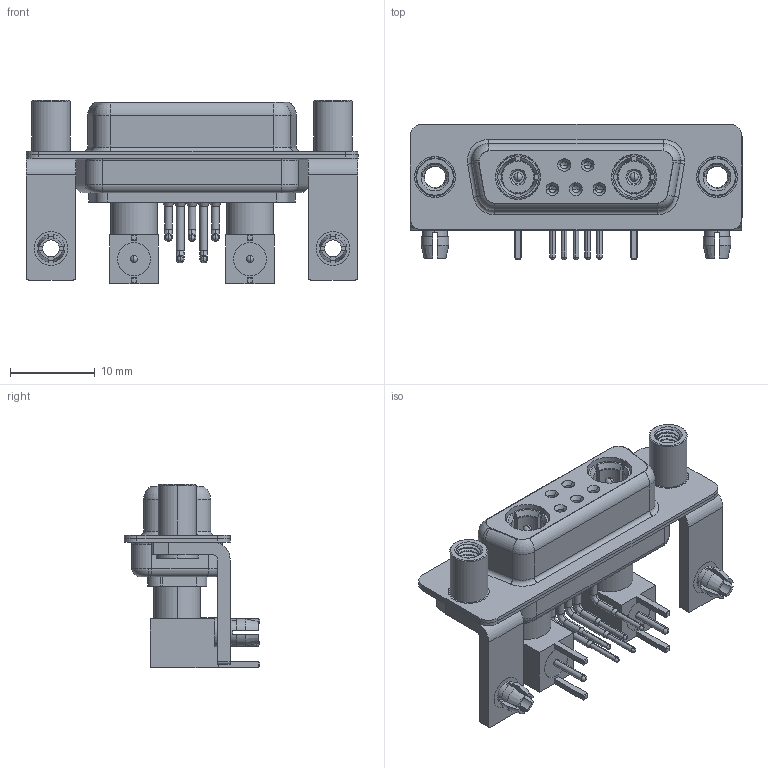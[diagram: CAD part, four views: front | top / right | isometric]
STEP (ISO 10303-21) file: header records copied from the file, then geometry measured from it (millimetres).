
FILE_DESCRIPTION (( 'STEP AP203' ), '1' );
FILE_NAME ('630-7W2-240-5ND.STEP', '2022-05-31T01:10:40', ( '' ), ( '' ), 'SwSTEP 2.0', 'SolidWorks 2020', '' );
FILE_SCHEMA (( 'CONFIG_CONTROL_DESIGN' ));
Length unit declared in the file: millimetre
Products named in the file (17): RA Back Shell; Pin_RA; Locking Collar; Insulator Pin_Straight PC Tail; Insulator RA Pin; 630Combo Contact Row 2; Co-Ax Plug Assy_RA; 630-7W2-240-5ND; 630Combo Threaded Standoff_D; 630Combo Stabilizer Bracket; Co-Ax Plug_RA PC Tail; 630Combo Shell Rear_15 Contacts; 630Combo Shell Front_15 Contacts; 630Combo Board Lock; 630Combo Housing_7W2; 630Combo Contact Row 1
Assembly tree (28 placements, depth 3):
  630-7W2-240-5ND
    630Combo Housing_7W2
    630Combo Shell Front_15 Contacts
    630Combo Shell Rear_15 Contacts
    630Combo Stabilizer Bracket  x2
    630Combo Board Lock  x2
    630Combo Threaded Standoff_D  x2
    Co-Ax Plug Assy_RA
      Co-Ax Plug_RA PC Tail
      Insulator Pin_Straight PC Tail
      Pin_RA
      Locking Collar
      RA Back Shell
      Insulator RA Pin
    Co-Ax Plug Assy_RA
      Co-Ax Plug_RA PC Tail
      Insulator Pin_Straight PC Tail
      Pin_RA
      Locking Collar
      RA Back Shell
      Insulator RA Pin
    630Combo Contact Row 1  x2
    630Combo Contact Row 2  x3
Bounding box: 39.2 x 16 x 21.61 mm (x, y, z)
Volume: 3393.1 mm3; surface area: 8460.6 mm2
Topology: 26 solids, 26 shells, 1070 faces, 2676 edges, 1692 vertices
Faces by surface type: cylinder 486, plane 346, cone 133, torus 69, bspline 28, sphere 8
Entity records: 24302 total; most frequent: CARTESIAN_POINT 6298, DIRECTION 3540, ORIENTED_EDGE 3216, EDGE_CURVE 1608, AXIS2_PLACEMENT_3D 1422, VERTEX_POINT 1025, EDGE_LOOP 749, CIRCLE 742
